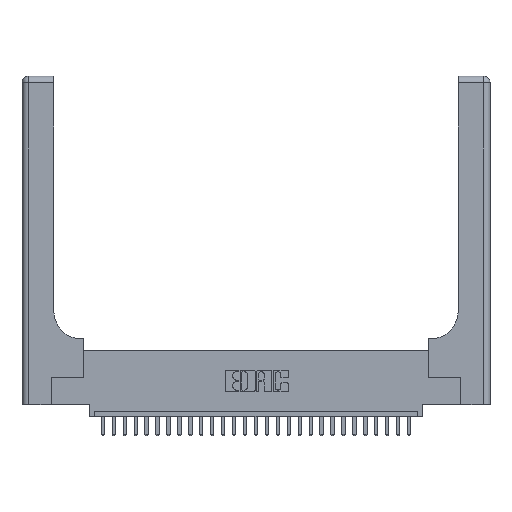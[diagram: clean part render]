
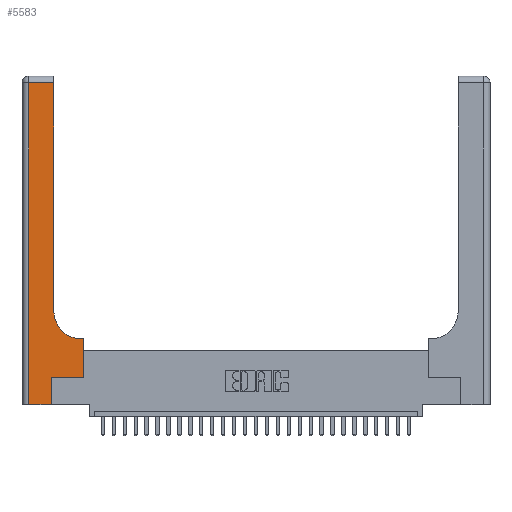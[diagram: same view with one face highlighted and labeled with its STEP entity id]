
A CAD part, top view. The second image highlights one B-rep face of the part: STEP entity #5583.
In plain terms, the highlighted planar face has unit normal (0, 0, 1).
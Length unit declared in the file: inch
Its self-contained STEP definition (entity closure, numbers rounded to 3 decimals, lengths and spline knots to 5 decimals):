
#851 = DIRECTION ( 'NONE',  ( 1., 0., 0. ) ) ;
#1093 = ORIENTED_EDGE ( 'NONE', *, *, #5474, .T. ) ;
#1607 = DIRECTION ( 'NONE',  ( 0., 1., 0. ) ) ;
#1925 = CARTESIAN_POINT ( 'NONE',  ( 0.5585, 0.6, 0.37 ) ) ;
#2666 = LINE ( 'NONE', #3727, #19159 ) ;
#2975 = CARTESIAN_POINT ( 'NONE',  ( 0.269, 0., 0.37 ) ) ;
#3062 = VECTOR ( 'NONE', #26009, 39.37008 ) ;
#3213 = DIRECTION ( 'NONE',  ( 0., 0., -1. ) ) ;
#3212 = CARTESIAN_POINT ( 'NONE',  ( 0.2915, 3., 0.37 ) ) ;
#3427 = DIRECTION ( 'NONE',  ( 0., 0., -1. ) ) ;
#3727 = CARTESIAN_POINT ( 'NONE',  ( 0.269, 0.25, 0.37 ) ) ;
#3822 = ORIENTED_EDGE ( 'NONE', *, *, #21351, .T. ) ;
#5474 = EDGE_CURVE ( 'NONE', #28385, #17374, #5968, .T. ) ;
#5534 = CARTESIAN_POINT ( 'NONE',  ( 0.5585, 0.25, 0.37 ) ) ;
#5583 = ADVANCED_FACE ( 'NONE', ( #21052 ), #21445, .F. ) ;
#5693 = VERTEX_POINT ( 'NONE', #1925 ) ;
#5743 = CARTESIAN_POINT ( 'NONE',  ( 0., 3., 0.37 ) ) ;
#5940 = DIRECTION ( 'NONE',  ( 1., 0., 0. ) ) ;
#5968 = CIRCLE ( 'NONE', #23219, 0.25 ) ;
#7114 = EDGE_CURVE ( 'NONE', #23752, #17583, #7617, .T. ) ;
#7596 = LINE ( 'NONE', #10688, #3062 ) ;
#7615 = CARTESIAN_POINT ( 'NONE',  ( 0.06, 3., 0.37 ) ) ;
#7617 = LINE ( 'NONE', #7615, #13895 ) ;
#8871 = ORIENTED_EDGE ( 'NONE', *, *, #23205, .T. ) ;
#8876 = CARTESIAN_POINT ( 'NONE',  ( 0.2915, 0.85, 0.37 ) ) ;
#10067 = ORIENTED_EDGE ( 'NONE', *, *, #26662, .T. ) ;
#10125 = LINE ( 'NONE', #12535, #22416 ) ;
#10688 = CARTESIAN_POINT ( 'NONE',  ( 0., 2.94, 0.37 ) ) ;
#11881 = CARTESIAN_POINT ( 'NONE',  ( 0.5415, 0.85, 0.37 ) ) ;
#12535 = CARTESIAN_POINT ( 'NONE',  ( 0.269, 0., 0.37 ) ) ;
#13139 = VECTOR ( 'NONE', #20799, 39.37008 ) ;
#13196 = EDGE_CURVE ( 'NONE', #5693, #28385, #14963, .T. ) ;
#13895 = VECTOR ( 'NONE', #28959, 39.37008 ) ;
#14477 = CARTESIAN_POINT ( 'NONE',  ( 0.2915, 0.6, 0.37 ) ) ;
#14963 = LINE ( 'NONE', #14477, #26213 ) ;
#15729 = LINE ( 'NONE', #3212, #24504 ) ;
#16483 = CARTESIAN_POINT ( 'NONE',  ( 0., 0., 0.37 ) ) ;
#17055 = VERTEX_POINT ( 'NONE', #19514 ) ;
#17304 = ORIENTED_EDGE ( 'NONE', *, *, #13196, .T. ) ;
#17374 = VERTEX_POINT ( 'NONE', #8876 ) ;
#17583 = VERTEX_POINT ( 'NONE', #28948 ) ;
#18724 = AXIS2_PLACEMENT_3D ( 'NONE', #5743, #3427, #25932 ) ;
#18882 = DIRECTION ( 'NONE',  ( 0., 1., 0. ) ) ;
#19159 = VECTOR ( 'NONE', #5940, 39.37008 ) ;
#19200 = CARTESIAN_POINT ( 'NONE',  ( 0.5585, 0.25, 0.37 ) ) ;
#19514 = CARTESIAN_POINT ( 'NONE',  ( 0.269, 0.25, 0.37 ) ) ;
#20091 = ORIENTED_EDGE ( 'NONE', *, *, #28288, .T. ) ;
#20327 = VERTEX_POINT ( 'NONE', #19200 ) ;
#20799 = DIRECTION ( 'NONE',  ( 0., 1., 0. ) ) ;
#20952 = ORIENTED_EDGE ( 'NONE', *, *, #20997, .T. ) ;
#20997 = EDGE_CURVE ( 'NONE', #17055, #20327, #2666, .T. ) ;
#21052 = FACE_OUTER_BOUND ( 'NONE', #21860, .T. ) ;
#21277 = DIRECTION ( 'NONE',  ( -1., 0., 0. ) ) ;
#21351 = EDGE_CURVE ( 'NONE', #20327, #5693, #26836, .T. ) ;
#21445 = PLANE ( 'NONE',  #18724 ) ;
#21444 = CARTESIAN_POINT ( 'NONE',  ( 0.5415, 0.6, 0.37 ) ) ;
#21860 = EDGE_LOOP ( 'NONE', ( #20091, #26398, #22024, #8871, #10067, #20952, #3822, #17304, #1093 ) ) ;
#21962 = VECTOR ( 'NONE', #27654, 39.37008 ) ;
#22024 = ORIENTED_EDGE ( 'NONE', *, *, #7114, .T. ) ;
#22117 = CARTESIAN_POINT ( 'NONE',  ( 0.2915, 2.94, 0.37 ) ) ;
#22416 = VECTOR ( 'NONE', #1607, 39.37008 ) ;
#23205 = EDGE_CURVE ( 'NONE', #17583, #24541, #23335, .T. ) ;
#23219 = AXIS2_PLACEMENT_3D ( 'NONE', #11881, #3213, #851 ) ;
#23335 = LINE ( 'NONE', #16483, #21962 ) ;
#23752 = VERTEX_POINT ( 'NONE', #27149 ) ;
#24504 = VECTOR ( 'NONE', #18882, 39.37008 ) ;
#24541 = VERTEX_POINT ( 'NONE', #2975 ) ;
#25932 = DIRECTION ( 'NONE',  ( -1., 0., 0. ) ) ;
#26009 = DIRECTION ( 'NONE',  ( -1., 0., 0. ) ) ;
#26213 = VECTOR ( 'NONE', #21277, 39.37008 ) ;
#26398 = ORIENTED_EDGE ( 'NONE', *, *, #28875, .T. ) ;
#26662 = EDGE_CURVE ( 'NONE', #24541, #17055, #10125, .T. ) ;
#26760 = VERTEX_POINT ( 'NONE', #22117 ) ;
#26836 = LINE ( 'NONE', #5534, #13139 ) ;
#27149 = CARTESIAN_POINT ( 'NONE',  ( 0.06, 2.94, 0.37 ) ) ;
#27654 = DIRECTION ( 'NONE',  ( 1., 0., 0. ) ) ;
#28288 = EDGE_CURVE ( 'NONE', #17374, #26760, #15729, .T. ) ;
#28385 = VERTEX_POINT ( 'NONE', #21444 ) ;
#28875 = EDGE_CURVE ( 'NONE', #26760, #23752, #7596, .T. ) ;
#28948 = CARTESIAN_POINT ( 'NONE',  ( 0.06, 0., 0.37 ) ) ;
#28959 = DIRECTION ( 'NONE',  ( 0., -1., 0. ) ) ;
